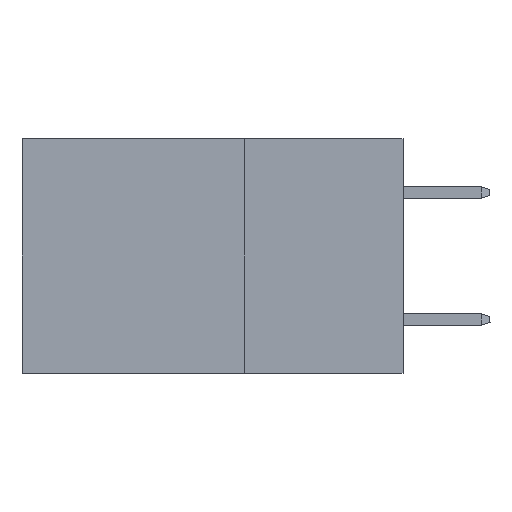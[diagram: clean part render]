
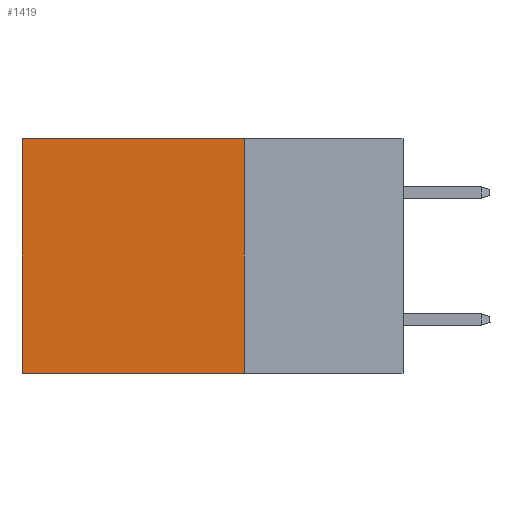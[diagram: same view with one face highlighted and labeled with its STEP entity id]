
A CAD part, left-side view. The second image highlights one B-rep face of the part: STEP entity #1419.
In plain terms, the highlighted planar face has unit normal (-1, 0, 0).
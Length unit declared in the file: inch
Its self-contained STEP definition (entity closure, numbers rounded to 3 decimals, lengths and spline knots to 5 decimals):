
#324 = PLANE ( 'NONE',  #6638 ) ;
#431 = VECTOR ( 'NONE', #4381, 39.37008 ) ;
#1157 = LINE ( 'NONE', #6804, #11238 ) ;
#1419 = ADVANCED_FACE ( 'NONE', ( #5985 ), #324, .F. ) ;
#1839 = VECTOR ( 'NONE', #10952, 39.37008 ) ;
#2000 = CARTESIAN_POINT ( 'NONE',  ( 0.2875, 0.25, 0. ) ) ;
#2178 = CARTESIAN_POINT ( 'NONE',  ( 0.2875, 0.6, 0. ) ) ;
#2946 = VECTOR ( 'NONE', #11305, 39.37008 ) ;
#4258 = EDGE_CURVE ( 'NONE', #10316, #11235, #7652, .T. ) ;
#4381 = DIRECTION ( 'NONE',  ( 0., 0., -1. ) ) ;
#4863 = VERTEX_POINT ( 'NONE', #5825 ) ;
#5825 = CARTESIAN_POINT ( 'NONE',  ( 0.2875, 0.6, 0. ) ) ;
#5985 = FACE_OUTER_BOUND ( 'NONE', #14527, .T. ) ;
#6517 = CARTESIAN_POINT ( 'NONE',  ( 0.2875, 0.6, -0.37 ) ) ;
#6638 = AXIS2_PLACEMENT_3D ( 'NONE', #8358, #10654, #7171 ) ;
#6804 = CARTESIAN_POINT ( 'NONE',  ( 0.2875, 0.25, 0. ) ) ;
#7171 = DIRECTION ( 'NONE',  ( 0., 0., -1. ) ) ;
#7553 = EDGE_CURVE ( 'NONE', #11235, #14356, #13282, .T. ) ;
#7652 = LINE ( 'NONE', #7728, #431 ) ;
#7728 = CARTESIAN_POINT ( 'NONE',  ( 0.2875, 0.25, 0. ) ) ;
#8239 = CARTESIAN_POINT ( 'NONE',  ( 0.2875, 0.25, -0.37 ) ) ;
#8358 = CARTESIAN_POINT ( 'NONE',  ( 0.2875, 0.25, 0. ) ) ;
#8599 = ORIENTED_EDGE ( 'NONE', *, *, #12376, .T. ) ;
#8934 = ORIENTED_EDGE ( 'NONE', *, *, #7553, .F. ) ;
#10222 = DIRECTION ( 'NONE',  ( 0., 1., 0. ) ) ;
#10316 = VERTEX_POINT ( 'NONE', #2000 ) ;
#10654 = DIRECTION ( 'NONE',  ( 1., 0., 0. ) ) ;
#10915 = ORIENTED_EDGE ( 'NONE', *, *, #13283, .T. ) ;
#10952 = DIRECTION ( 'NONE',  ( 0., 1., 0. ) ) ;
#11235 = VERTEX_POINT ( 'NONE', #8239 ) ;
#11238 = VECTOR ( 'NONE', #10222, 39.37008 ) ;
#11305 = DIRECTION ( 'NONE',  ( 0., 0., -1. ) ) ;
#12157 = CARTESIAN_POINT ( 'NONE',  ( 0.2875, 0.25, -0.37 ) ) ;
#12357 = LINE ( 'NONE', #2178, #2946 ) ;
#12376 = EDGE_CURVE ( 'NONE', #4863, #14356, #12357, .T. ) ;
#13282 = LINE ( 'NONE', #12157, #1839 ) ;
#13283 = EDGE_CURVE ( 'NONE', #10316, #4863, #1157, .T. ) ;
#14236 = ORIENTED_EDGE ( 'NONE', *, *, #4258, .F. ) ;
#14356 = VERTEX_POINT ( 'NONE', #6517 ) ;
#14527 = EDGE_LOOP ( 'NONE', ( #8599, #8934, #14236, #10915 ) ) ;
